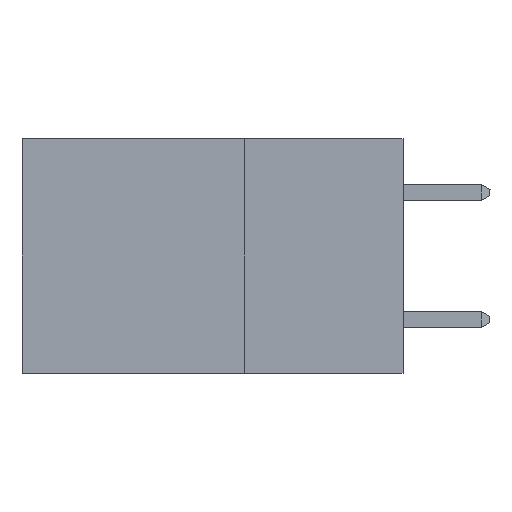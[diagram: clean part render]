
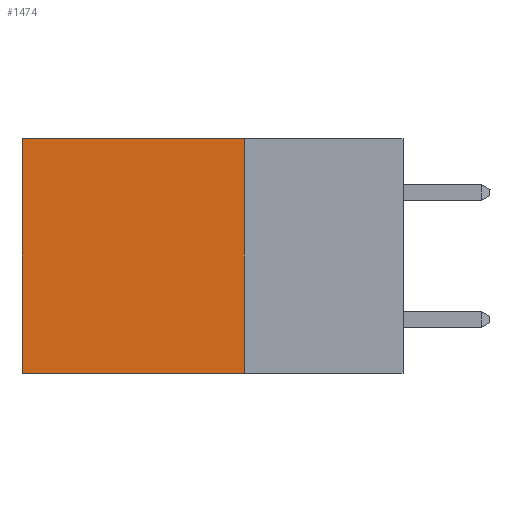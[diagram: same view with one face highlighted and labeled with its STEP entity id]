
A CAD part, left-side view. The second image highlights one B-rep face of the part: STEP entity #1474.
In plain terms, the highlighted planar face has unit normal (-1, 0, 0).
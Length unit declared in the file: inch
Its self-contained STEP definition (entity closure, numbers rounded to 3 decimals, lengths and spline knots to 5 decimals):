
#17 = LINE ( 'NONE', #5746, #8299 ) ;
#116 = VERTEX_POINT ( 'NONE', #7018 ) ;
#556 = CARTESIAN_POINT ( 'NONE',  ( 0.2875, 0.25, 0. ) ) ;
#602 = CARTESIAN_POINT ( 'NONE',  ( 0.2875, 0.25, 0. ) ) ;
#704 = DIRECTION ( 'NONE',  ( 0., 0., -1. ) ) ;
#880 = DIRECTION ( 'NONE',  ( 1., 0., 0. ) ) ;
#1051 = EDGE_CURVE ( 'NONE', #116, #11015, #12530, .T. ) ;
#1474 = ADVANCED_FACE ( 'NONE', ( #13484 ), #5153, .F. ) ;
#1482 = LINE ( 'NONE', #11534, #9580 ) ;
#2534 = VERTEX_POINT ( 'NONE', #3234 ) ;
#3234 = CARTESIAN_POINT ( 'NONE',  ( 0.2875, 0.6, 0. ) ) ;
#3354 = CARTESIAN_POINT ( 'NONE',  ( 0.2875, 0.25, -0.37 ) ) ;
#3372 = VECTOR ( 'NONE', #10173, 39.37008 ) ;
#3739 = EDGE_LOOP ( 'NONE', ( #5809, #5825, #5980, #6041 ) ) ;
#4076 = DIRECTION ( 'NONE',  ( 0., 1., 0. ) ) ;
#4383 = DIRECTION ( 'NONE',  ( 0., 1., 0. ) ) ;
#5153 = PLANE ( 'NONE',  #8863 ) ;
#5448 = EDGE_CURVE ( 'NONE', #9680, #2534, #1482, .T. ) ;
#5581 = CARTESIAN_POINT ( 'NONE',  ( 0.2875, 0.25, 0. ) ) ;
#5746 = CARTESIAN_POINT ( 'NONE',  ( 0.2875, 0.6, 0. ) ) ;
#5809 = ORIENTED_EDGE ( 'NONE', *, *, #8676, .T. ) ;
#5825 = ORIENTED_EDGE ( 'NONE', *, *, #1051, .F. ) ;
#5980 = ORIENTED_EDGE ( 'NONE', *, *, #9710, .F. ) ;
#6041 = ORIENTED_EDGE ( 'NONE', *, *, #5448, .T. ) ;
#6132 = LINE ( 'NONE', #602, #3372 ) ;
#7018 = CARTESIAN_POINT ( 'NONE',  ( 0.2875, 0.25, -0.37 ) ) ;
#7208 = VECTOR ( 'NONE', #4076, 39.37008 ) ;
#8299 = VECTOR ( 'NONE', #11884, 39.37008 ) ;
#8676 = EDGE_CURVE ( 'NONE', #2534, #11015, #17, .T. ) ;
#8863 = AXIS2_PLACEMENT_3D ( 'NONE', #5581, #880, #704 ) ;
#9580 = VECTOR ( 'NONE', #4383, 39.37008 ) ;
#9680 = VERTEX_POINT ( 'NONE', #556 ) ;
#9710 = EDGE_CURVE ( 'NONE', #9680, #116, #6132, .T. ) ;
#10173 = DIRECTION ( 'NONE',  ( 0., 0., -1. ) ) ;
#11015 = VERTEX_POINT ( 'NONE', #12009 ) ;
#11534 = CARTESIAN_POINT ( 'NONE',  ( 0.2875, 0.25, 0. ) ) ;
#11884 = DIRECTION ( 'NONE',  ( 0., 0., -1. ) ) ;
#12009 = CARTESIAN_POINT ( 'NONE',  ( 0.2875, 0.6, -0.37 ) ) ;
#12530 = LINE ( 'NONE', #3354, #7208 ) ;
#13484 = FACE_OUTER_BOUND ( 'NONE', #3739, .T. ) ;
